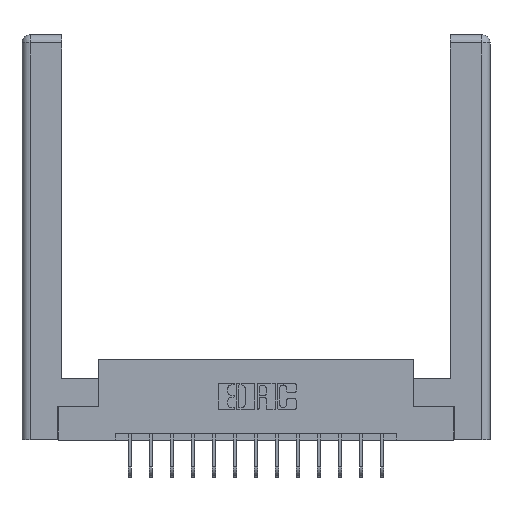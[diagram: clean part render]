
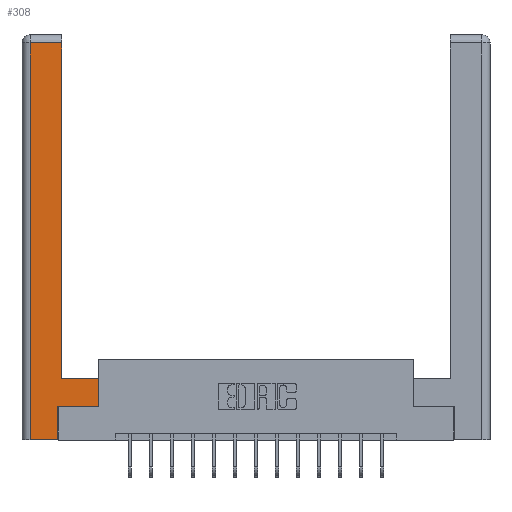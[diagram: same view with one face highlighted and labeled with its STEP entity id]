
A CAD part, top view. The second image highlights one B-rep face of the part: STEP entity #308.
In plain terms, the highlighted planar face has unit normal (0, 0, 1).
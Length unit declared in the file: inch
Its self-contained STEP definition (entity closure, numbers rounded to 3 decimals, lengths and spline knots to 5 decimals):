
#194 = ORIENTED_EDGE ( 'NONE', *, *, #8309, .T. ) ;
#308 = ADVANCED_FACE ( 'NONE', ( #17433 ), #6015, .F. ) ;
#316 = VECTOR ( 'NONE', #16893, 39.37008 ) ;
#408 = CARTESIAN_POINT ( 'NONE',  ( 0.0615, 2.94, 0. ) ) ;
#431 = DIRECTION ( 'NONE',  ( -1., 0., 0. ) ) ;
#449 = DIRECTION ( 'NONE',  ( 0., 1., 0. ) ) ;
#485 = VECTOR ( 'NONE', #896, 39.37008 ) ;
#624 = LINE ( 'NONE', #9569, #14768 ) ;
#865 = CARTESIAN_POINT ( 'NONE',  ( 0.565, 0.245, 0. ) ) ;
#896 = DIRECTION ( 'NONE',  ( 0., 1., 0. ) ) ;
#2433 = DIRECTION ( 'NONE',  ( -1., 0., 0. ) ) ;
#2631 = CARTESIAN_POINT ( 'NONE',  ( 0.265, 0., 0. ) ) ;
#3187 = CARTESIAN_POINT ( 'NONE',  ( 0.265, 0.245, 0. ) ) ;
#3609 = EDGE_CURVE ( 'NONE', #17719, #7092, #16641, .T. ) ;
#3916 = ORIENTED_EDGE ( 'NONE', *, *, #11083, .T. ) ;
#3928 = DIRECTION ( 'NONE',  ( 1., 0., 0. ) ) ;
#4080 = CARTESIAN_POINT ( 'NONE',  ( 0.265, 0., 0. ) ) ;
#4471 = LINE ( 'NONE', #6690, #485 ) ;
#4507 = VERTEX_POINT ( 'NONE', #865 ) ;
#4640 = CARTESIAN_POINT ( 'NONE',  ( 0.265, 0.245, 0. ) ) ;
#5301 = EDGE_CURVE ( 'NONE', #12685, #17719, #11100, .T. ) ;
#5566 = CARTESIAN_POINT ( 'NONE',  ( 0.295, 0.45, 0. ) ) ;
#5699 = EDGE_CURVE ( 'NONE', #7092, #17651, #16591, .T. ) ;
#5758 = DIRECTION ( 'NONE',  ( 0., 1., 0. ) ) ;
#5829 = DIRECTION ( 'NONE',  ( 0., 0., -1. ) ) ;
#6015 = PLANE ( 'NONE',  #12612 ) ;
#6035 = CARTESIAN_POINT ( 'NONE',  ( 0.295, 3., 0. ) ) ;
#6083 = ORIENTED_EDGE ( 'NONE', *, *, #3609, .T. ) ;
#6170 = EDGE_CURVE ( 'NONE', #11247, #12685, #6949, .T. ) ;
#6450 = ORIENTED_EDGE ( 'NONE', *, *, #5301, .T. ) ;
#6546 = CARTESIAN_POINT ( 'NONE',  ( 0.0615, 0., 0. ) ) ;
#6690 = CARTESIAN_POINT ( 'NONE',  ( 0.565, 0.45, 0. ) ) ;
#6949 = LINE ( 'NONE', #6035, #8284 ) ;
#7092 = VERTEX_POINT ( 'NONE', #6546 ) ;
#7111 = VECTOR ( 'NONE', #7528, 39.37008 ) ;
#7528 = DIRECTION ( 'NONE',  ( -1., 0., 0. ) ) ;
#8048 = VECTOR ( 'NONE', #5758, 39.37008 ) ;
#8284 = VECTOR ( 'NONE', #449, 39.37008 ) ;
#8309 = EDGE_CURVE ( 'NONE', #4507, #17576, #4471, .T. ) ;
#8405 = EDGE_CURVE ( 'NONE', #17576, #11247, #10221, .T. ) ;
#8464 = VECTOR ( 'NONE', #13784, 39.37008 ) ;
#9167 = VERTEX_POINT ( 'NONE', #4640 ) ;
#9569 = CARTESIAN_POINT ( 'NONE',  ( 0.565, 0.245, 0. ) ) ;
#10221 = LINE ( 'NONE', #15055, #16797 ) ;
#10729 = ORIENTED_EDGE ( 'NONE', *, *, #8405, .T. ) ;
#10861 = ORIENTED_EDGE ( 'NONE', *, *, #5699, .T. ) ;
#11018 = CARTESIAN_POINT ( 'NONE',  ( 0.0615, 2.94, 0. ) ) ;
#11083 = EDGE_CURVE ( 'NONE', #9167, #4507, #624, .T. ) ;
#11100 = LINE ( 'NONE', #408, #7111 ) ;
#11247 = VERTEX_POINT ( 'NONE', #5566 ) ;
#11857 = EDGE_LOOP ( 'NONE', ( #16092, #6450, #6083, #10861, #13279, #3916, #194, #10729 ) ) ;
#12612 = AXIS2_PLACEMENT_3D ( 'NONE', #17323, #5829, #431 ) ;
#12685 = VERTEX_POINT ( 'NONE', #14576 ) ;
#12786 = CARTESIAN_POINT ( 'NONE',  ( 0.0615, 0., 0. ) ) ;
#13279 = ORIENTED_EDGE ( 'NONE', *, *, #16399, .T. ) ;
#13784 = DIRECTION ( 'NONE',  ( 1., 0., 0. ) ) ;
#14576 = CARTESIAN_POINT ( 'NONE',  ( 0.295, 2.94, 0. ) ) ;
#14768 = VECTOR ( 'NONE', #3928, 39.37008 ) ;
#15055 = CARTESIAN_POINT ( 'NONE',  ( 0.295, 0.45, 0. ) ) ;
#15536 = LINE ( 'NONE', #3187, #8048 ) ;
#16092 = ORIENTED_EDGE ( 'NONE', *, *, #6170, .T. ) ;
#16399 = EDGE_CURVE ( 'NONE', #17651, #9167, #15536, .T. ) ;
#16591 = LINE ( 'NONE', #2631, #8464 ) ;
#16641 = LINE ( 'NONE', #12786, #316 ) ;
#16797 = VECTOR ( 'NONE', #2433, 39.37008 ) ;
#16893 = DIRECTION ( 'NONE',  ( 0., -1., 0. ) ) ;
#17323 = CARTESIAN_POINT ( 'NONE',  ( 0., 0., 0. ) ) ;
#17433 = FACE_OUTER_BOUND ( 'NONE', #11857, .T. ) ;
#17576 = VERTEX_POINT ( 'NONE', #17794 ) ;
#17651 = VERTEX_POINT ( 'NONE', #4080 ) ;
#17719 = VERTEX_POINT ( 'NONE', #11018 ) ;
#17794 = CARTESIAN_POINT ( 'NONE',  ( 0.565, 0.45, 0. ) ) ;
